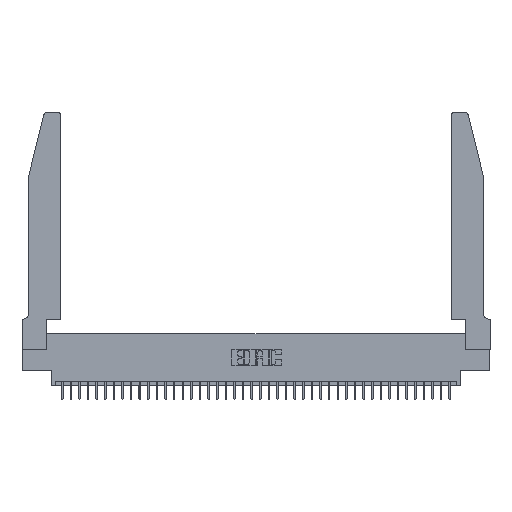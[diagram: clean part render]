
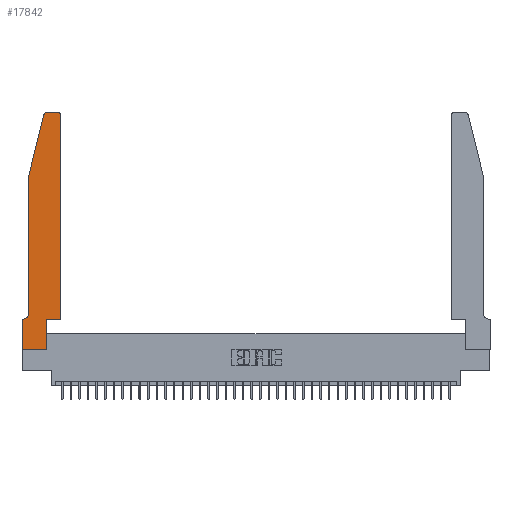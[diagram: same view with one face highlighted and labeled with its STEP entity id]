
A CAD part, top view. The second image highlights one B-rep face of the part: STEP entity #17842.
In plain terms, the highlighted planar face has unit normal (0, 0, 1).
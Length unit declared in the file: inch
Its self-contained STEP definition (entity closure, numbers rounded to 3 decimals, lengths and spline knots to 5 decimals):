
#2 = EDGE_CURVE ( 'NONE', #6956, #10742, #426, .T. ) ;
#426 = CIRCLE ( 'NONE', #1702, 0.03 ) ;
#564 = DIRECTION ( 'NONE',  ( 1., 0., 0. ) ) ;
#1702 = AXIS2_PLACEMENT_3D ( 'NONE', #16243, #38124, #564 ) ;
#2060 = ORIENTED_EDGE ( 'NONE', *, *, #9456, .T. ) ;
#2272 = ORIENTED_EDGE ( 'NONE', *, *, #23438, .T. ) ;
#3142 = CARTESIAN_POINT ( 'NONE',  ( 0., 0., 0.37 ) ) ;
#3767 = CARTESIAN_POINT ( 'NONE',  ( 0.4505, 0.35, 0.37 ) ) ;
#4353 = CARTESIAN_POINT ( 'NONE',  ( 0.284, 2.75, 0.37 ) ) ;
#4627 = ORIENTED_EDGE ( 'NONE', *, *, #28644, .T. ) ;
#4819 = CARTESIAN_POINT ( 'NONE',  ( 0.4505, 0.35, 0.37 ) ) ;
#4966 = CARTESIAN_POINT ( 'NONE',  ( 0.4505, 2.72, 0.37 ) ) ;
#5491 = FACE_OUTER_BOUND ( 'NONE', #26712, .T. ) ;
#5723 = DIRECTION ( 'NONE',  ( -1., 0., 0. ) ) ;
#5925 = LINE ( 'NONE', #32890, #19695 ) ;
#6005 = LINE ( 'NONE', #21551, #20780 ) ;
#6664 = AXIS2_PLACEMENT_3D ( 'NONE', #23169, #20021, #29611 ) ;
#6956 = VERTEX_POINT ( 'NONE', #4966 ) ;
#8378 = VERTEX_POINT ( 'NONE', #18759 ) ;
#8711 = CARTESIAN_POINT ( 'NONE',  ( 0., 0.35, 0.37 ) ) ;
#9456 = EDGE_CURVE ( 'NONE', #23957, #8378, #13905, .T. ) ;
#10052 = ORIENTED_EDGE ( 'NONE', *, *, #12524, .T. ) ;
#10742 = VERTEX_POINT ( 'NONE', #11015 ) ;
#11015 = CARTESIAN_POINT ( 'NONE',  ( 0.4205, 2.75, 0.37 ) ) ;
#11095 = VECTOR ( 'NONE', #31706, 39.37008 ) ;
#12464 = CARTESIAN_POINT ( 'NONE',  ( 0.0755, 0.42, 0.37 ) ) ;
#12524 = EDGE_CURVE ( 'NONE', #29016, #27014, #14700, .T. ) ;
#13486 = CARTESIAN_POINT ( 'NONE',  ( 0.2605, 2.75, 0.37 ) ) ;
#13744 = DIRECTION ( 'NONE',  ( -0.239, -0.971, 0. ) ) ;
#13805 = DIRECTION ( 'NONE',  ( 0., -1., 0. ) ) ;
#13829 = EDGE_CURVE ( 'NONE', #27014, #22073, #40061, .T. ) ;
#13905 = CIRCLE ( 'NONE', #24052, 0.07 ) ;
#14096 = VECTOR ( 'NONE', #39397, 39.37008 ) ;
#14697 = ORIENTED_EDGE ( 'NONE', *, *, #2, .T. ) ;
#14700 = CIRCLE ( 'NONE', #6664, 0.03 ) ;
#15590 = CARTESIAN_POINT ( 'NONE',  ( 0.2865, 0.35, 0.37 ) ) ;
#16243 = CARTESIAN_POINT ( 'NONE',  ( 0.4205, 2.72, 0.37 ) ) ;
#17469 = DIRECTION ( 'NONE',  ( 1., 0., 0. ) ) ;
#17545 = CARTESIAN_POINT ( 'NONE',  ( 0.0755, 0.35, 0.37 ) ) ;
#17842 = ADVANCED_FACE ( 'NONE', ( #5491 ), #39069, .T. ) ;
#18164 = LINE ( 'NONE', #4819, #23561 ) ;
#18622 = EDGE_CURVE ( 'NONE', #29374, #31771, #5925, .T. ) ;
#18759 = CARTESIAN_POINT ( 'NONE',  ( 0.0055, 0.35, 0.37 ) ) ;
#18893 = ORIENTED_EDGE ( 'NONE', *, *, #22800, .T. ) ;
#19081 = LINE ( 'NONE', #13486, #25934 ) ;
#19115 = LINE ( 'NONE', #15590, #30884 ) ;
#19695 = VECTOR ( 'NONE', #13805, 39.37008 ) ;
#20021 = DIRECTION ( 'NONE',  ( 0., 0., 1. ) ) ;
#20035 = DIRECTION ( 'NONE',  ( 1., 0., 0. ) ) ;
#20309 = CARTESIAN_POINT ( 'NONE',  ( 0., 0., 0.37 ) ) ;
#20481 = VECTOR ( 'NONE', #13744, 39.37008 ) ;
#20622 = CARTESIAN_POINT ( 'NONE',  ( 0.2865, 0., 0.37 ) ) ;
#20677 = EDGE_CURVE ( 'NONE', #8378, #29374, #30814, .T. ) ;
#20780 = VECTOR ( 'NONE', #21682, 39.37008 ) ;
#21551 = CARTESIAN_POINT ( 'NONE',  ( 0.0755, 2., 0.37 ) ) ;
#21682 = DIRECTION ( 'NONE',  ( 0., -1., 0. ) ) ;
#21763 = ORIENTED_EDGE ( 'NONE', *, *, #37646, .T. ) ;
#22073 = VERTEX_POINT ( 'NONE', #25759 ) ;
#22176 = VERTEX_POINT ( 'NONE', #35604 ) ;
#22543 = EDGE_CURVE ( 'NONE', #30896, #22176, #19115, .T. ) ;
#22800 = EDGE_CURVE ( 'NONE', #10742, #29016, #19081, .T. ) ;
#23169 = CARTESIAN_POINT ( 'NONE',  ( 0.284, 2.72, 0.37 ) ) ;
#23438 = EDGE_CURVE ( 'NONE', #28006, #6956, #38535, .T. ) ;
#23561 = VECTOR ( 'NONE', #17469, 39.37008 ) ;
#23957 = VERTEX_POINT ( 'NONE', #12464 ) ;
#24052 = AXIS2_PLACEMENT_3D ( 'NONE', #24568, #30436, #5723 ) ;
#24568 = CARTESIAN_POINT ( 'NONE',  ( 0.0055, 0.42, 0.37 ) ) ;
#25632 = VECTOR ( 'NONE', #20035, 39.37008 ) ;
#25759 = CARTESIAN_POINT ( 'NONE',  ( 0.0755, 2., 0.37 ) ) ;
#25934 = VECTOR ( 'NONE', #25991, 39.37008 ) ;
#25991 = DIRECTION ( 'NONE',  ( -1., 0., 0. ) ) ;
#26072 = ORIENTED_EDGE ( 'NONE', *, *, #20677, .T. ) ;
#26712 = EDGE_LOOP ( 'NONE', ( #18893, #10052, #29733, #31540, #2060, #26072, #27770, #21763, #35472, #4627, #2272, #14697 ) ) ;
#27014 = VERTEX_POINT ( 'NONE', #35006 ) ;
#27770 = ORIENTED_EDGE ( 'NONE', *, *, #18622, .T. ) ;
#28006 = VERTEX_POINT ( 'NONE', #3767 ) ;
#28644 = EDGE_CURVE ( 'NONE', #22176, #28006, #18164, .T. ) ;
#28981 = CARTESIAN_POINT ( 'NONE',  ( 0.4505, 0.35, 0.37 ) ) ;
#29016 = VERTEX_POINT ( 'NONE', #4353 ) ;
#29374 = VERTEX_POINT ( 'NONE', #8711 ) ;
#29611 = DIRECTION ( 'NONE',  ( 1., 0., 0. ) ) ;
#29733 = ORIENTED_EDGE ( 'NONE', *, *, #13829, .T. ) ;
#30082 = AXIS2_PLACEMENT_3D ( 'NONE', #38653, #38781, #32959 ) ;
#30436 = DIRECTION ( 'NONE',  ( 0., 0., -1. ) ) ;
#30814 = LINE ( 'NONE', #17545, #14096 ) ;
#30884 = VECTOR ( 'NONE', #34258, 39.37008 ) ;
#30896 = VERTEX_POINT ( 'NONE', #20622 ) ;
#31540 = ORIENTED_EDGE ( 'NONE', *, *, #36528, .T. ) ;
#31706 = DIRECTION ( 'NONE',  ( 0., 1., 0. ) ) ;
#31771 = VERTEX_POINT ( 'NONE', #3142 ) ;
#32890 = CARTESIAN_POINT ( 'NONE',  ( 0., 0., 0.37 ) ) ;
#32959 = DIRECTION ( 'NONE',  ( 1., 0., 0. ) ) ;
#32984 = LINE ( 'NONE', #20309, #25632 ) ;
#34258 = DIRECTION ( 'NONE',  ( 0., 1., 0. ) ) ;
#35006 = CARTESIAN_POINT ( 'NONE',  ( 0.25487, 2.72718, 0.37 ) ) ;
#35472 = ORIENTED_EDGE ( 'NONE', *, *, #22543, .T. ) ;
#35604 = CARTESIAN_POINT ( 'NONE',  ( 0.2865, 0.35, 0.37 ) ) ;
#36528 = EDGE_CURVE ( 'NONE', #22073, #23957, #6005, .T. ) ;
#37646 = EDGE_CURVE ( 'NONE', #31771, #30896, #32984, .T. ) ;
#38124 = DIRECTION ( 'NONE',  ( 0., 0., 1. ) ) ;
#38535 = LINE ( 'NONE', #28981, #11095 ) ;
#38653 = CARTESIAN_POINT ( 'NONE',  ( 0., 0.35, 0.37 ) ) ;
#38781 = DIRECTION ( 'NONE',  ( 0., 0., 1. ) ) ;
#39065 = CARTESIAN_POINT ( 'NONE',  ( 0.0755, 2., 0.37 ) ) ;
#39069 = PLANE ( 'NONE',  #30082 ) ;
#39397 = DIRECTION ( 'NONE',  ( -1., 0., 0. ) ) ;
#40061 = LINE ( 'NONE', #39065, #20481 ) ;
